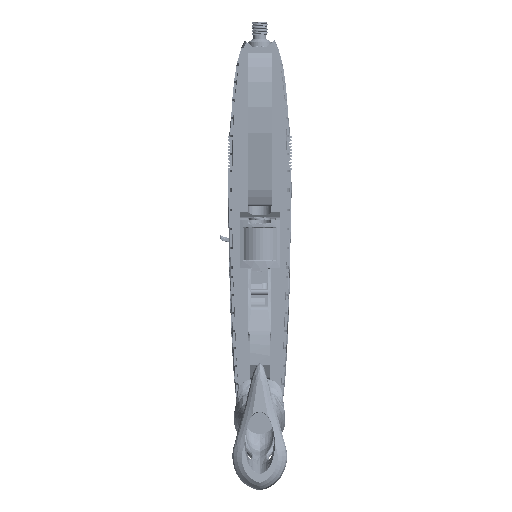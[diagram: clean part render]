
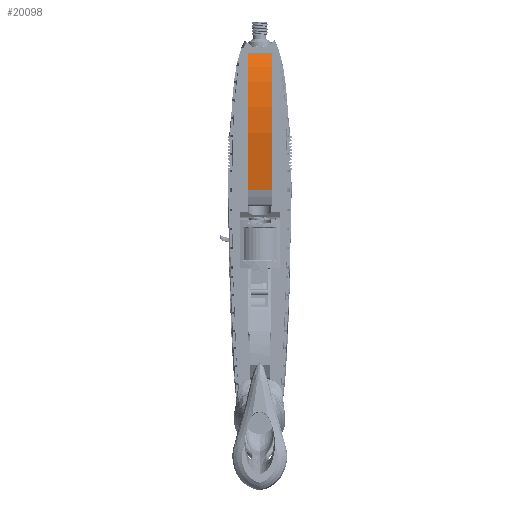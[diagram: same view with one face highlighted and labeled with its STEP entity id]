
A CAD part, front view. The second image highlights one B-rep face of the part: STEP entity #20098.
In plain terms, the highlighted free-form (B-spline) face has degree [7, 1] with [8, 2] control points.
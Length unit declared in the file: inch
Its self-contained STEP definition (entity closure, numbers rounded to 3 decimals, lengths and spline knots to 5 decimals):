
#332 = CARTESIAN_POINT ( 'NONE',  ( 0.254, -2.74429, 2.33483 ) ) ;
#930 = B_SPLINE_CURVE_WITH_KNOTS ( 'NONE', 7,
 ( #164528, #132977, #162384, #48482, #15977, #165599, #179708, #13831 ),
 .UNSPECIFIED., .F., .F.,
 ( 8, 8 ),
 ( 0., 1. ),
 .UNSPECIFIED. ) ;
#7942 = CARTESIAN_POINT ( 'NONE',  ( 1.004, -2.40554, 0. ) ) ;
#9030 = CARTESIAN_POINT ( 'NONE',  ( 1.004, -2.5891, 3.54336 ) ) ;
#13404 = CARTESIAN_POINT ( 'NONE',  ( 1.004, -2.15756, 4.32504 ) ) ;
#13831 = CARTESIAN_POINT ( 'NONE',  ( 0.254, -2.15756, 4.32504 ) ) ;
#14982 = ORIENTED_EDGE ( 'NONE', *, *, #119688, .T. ) ;
#15545 = FACE_OUTER_BOUND ( 'NONE', #196146, .T. ) ;
#15977 = CARTESIAN_POINT ( 'NONE',  ( 0.254, -2.72271, 3.06516 ) ) ;
#16608 = CARTESIAN_POINT ( 'NONE',  ( 0.254, -2.66061, 1.54519 ) ) ;
#20098 = ADVANCED_FACE ( 'NONE', ( #15545 ), #128084, .F. ) ;
#27902 = LINE ( 'NONE', #128711, #51987 ) ;
#29001 = DIRECTION ( 'NONE',  ( 1., 0., 0. ) ) ;
#29673 = CARTESIAN_POINT ( 'NONE',  ( 0.254, -2.15756, 4.32504 ) ) ;
#34702 = VERTEX_POINT ( 'NONE', #102743 ) ;
#35822 = VERTEX_POINT ( 'NONE', #198569 ) ;
#41546 = CARTESIAN_POINT ( 'NONE',  ( 1.004, -2.72271, 3.06516 ) ) ;
#47005 = CARTESIAN_POINT ( 'NONE',  ( 1.004, -2.55616, 0.77053 ) ) ;
#48482 = CARTESIAN_POINT ( 'NONE',  ( 0.254, -2.74429, 2.33483 ) ) ;
#51987 = VECTOR ( 'NONE', #29001, 39.37008 ) ;
#68474 = DIRECTION ( 'NONE',  ( 1., 0., 0. ) ) ;
#73048 = CARTESIAN_POINT ( 'NONE',  ( 1.004, -2.74429, 2.33483 ) ) ;
#75187 = CARTESIAN_POINT ( 'NONE',  ( 1.004, -2.36869, 4.11498 ) ) ;
#80634 = CARTESIAN_POINT ( 'NONE',  ( 0.254, -2.5891, 3.54336 ) ) ;
#82742 = CARTESIAN_POINT ( 'NONE',  ( 1.004, -2.74429, 2.33483 ) ) ;
#88263 = CARTESIAN_POINT ( 'NONE',  ( 1.004, -2.15756, 4.32504 ) ) ;
#89322 = CARTESIAN_POINT ( 'NONE',  ( 1.004, -2.66061, 1.54519 ) ) ;
#94705 = CARTESIAN_POINT ( 'NONE',  ( 1.004, -2.36869, 4.11498 ) ) ;
#102743 = CARTESIAN_POINT ( 'NONE',  ( 0.254, -2.15756, 4.32504 ) ) ;
#112099 = CARTESIAN_POINT ( 'NONE',  ( 0.254, -2.72271, 3.06516 ) ) ;
#116210 = EDGE_CURVE ( 'NONE', #35822, #34702, #930, .T. ) ;
#119688 = EDGE_CURVE ( 'NONE', #35822, #198576, #27902, .T. ) ;
#121929 = EDGE_CURVE ( 'NONE', #198576, #189627, #146802, .T. ) ;
#128084 = B_SPLINE_SURFACE_WITH_KNOTS ( 'NONE', 7, 1, ( 
 ( #210826, #197740 ),
 ( #211885, #47005 ),
 ( #16608, #147815 ),
 ( #332, #82742 ),
 ( #112099, #148866 ),
 ( #80634, #161959 ),
 ( #144588, #94705 ),
 ( #29673, #13404 ) ),
 .UNSPECIFIED., .F., .F., .F.,
 ( 8, 8 ),
 ( 2, 2 ),
 ( 0., 1. ),
 ( 0., 1. ),
 .UNSPECIFIED. ) ;
#128711 = CARTESIAN_POINT ( 'NONE',  ( 0.254, -2.40554, 0. ) ) ;
#132977 = CARTESIAN_POINT ( 'NONE',  ( 0.254, -2.55616, 0.77053 ) ) ;
#139131 = CARTESIAN_POINT ( 'NONE',  ( 1.004, -2.55616, 0.77053 ) ) ;
#139455 = EDGE_CURVE ( 'NONE', #34702, #189627, #168207, .T. ) ;
#139946 = CARTESIAN_POINT ( 'NONE',  ( 1.004, -2.15756, 4.32504 ) ) ;
#144588 = CARTESIAN_POINT ( 'NONE',  ( 0.254, -2.36869, 4.11498 ) ) ;
#146802 = B_SPLINE_CURVE_WITH_KNOTS ( 'NONE', 7,
 ( #7942, #139131, #89322, #73048, #41546, #9030, #75187, #88263 ),
 .UNSPECIFIED., .F., .F.,
 ( 8, 8 ),
 ( 0., 1. ),
 .UNSPECIFIED. ) ;
#147815 = CARTESIAN_POINT ( 'NONE',  ( 1.004, -2.66061, 1.54519 ) ) ;
#148866 = CARTESIAN_POINT ( 'NONE',  ( 1.004, -2.72271, 3.06516 ) ) ;
#150393 = CARTESIAN_POINT ( 'NONE',  ( 1.004, -2.40554, 0. ) ) ;
#161959 = CARTESIAN_POINT ( 'NONE',  ( 1.004, -2.5891, 3.54336 ) ) ;
#162384 = CARTESIAN_POINT ( 'NONE',  ( 0.254, -2.66061, 1.54519 ) ) ;
#164528 = CARTESIAN_POINT ( 'NONE',  ( 0.254, -2.40554, 0. ) ) ;
#165599 = CARTESIAN_POINT ( 'NONE',  ( 0.254, -2.5891, 3.54336 ) ) ;
#168207 = LINE ( 'NONE', #198656, #202154 ) ;
#171525 = ORIENTED_EDGE ( 'NONE', *, *, #139455, .F. ) ;
#174239 = ORIENTED_EDGE ( 'NONE', *, *, #116210, .F. ) ;
#179708 = CARTESIAN_POINT ( 'NONE',  ( 0.254, -2.36869, 4.11498 ) ) ;
#189627 = VERTEX_POINT ( 'NONE', #139946 ) ;
#196146 = EDGE_LOOP ( 'NONE', ( #206795, #171525, #174239, #14982 ) ) ;
#197740 = CARTESIAN_POINT ( 'NONE',  ( 1.004, -2.40554, 0. ) ) ;
#198569 = CARTESIAN_POINT ( 'NONE',  ( 0.254, -2.40554, 0. ) ) ;
#198576 = VERTEX_POINT ( 'NONE', #150393 ) ;
#198656 = CARTESIAN_POINT ( 'NONE',  ( 0.254, -2.15756, 4.32504 ) ) ;
#202154 = VECTOR ( 'NONE', #68474, 39.37008 ) ;
#206795 = ORIENTED_EDGE ( 'NONE', *, *, #121929, .T. ) ;
#210826 = CARTESIAN_POINT ( 'NONE',  ( 0.254, -2.40554, 0. ) ) ;
#211885 = CARTESIAN_POINT ( 'NONE',  ( 0.254, -2.55616, 0.77053 ) ) ;
